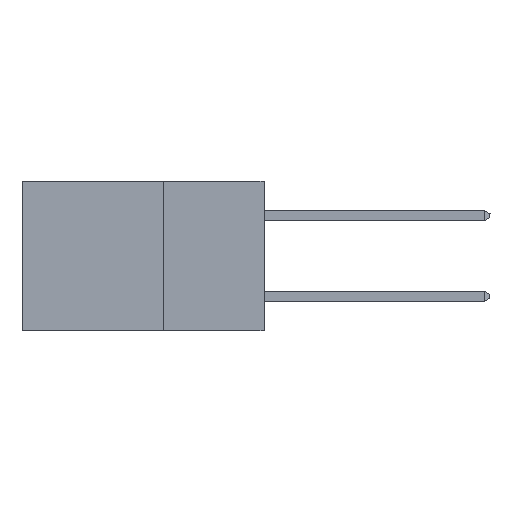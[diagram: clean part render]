
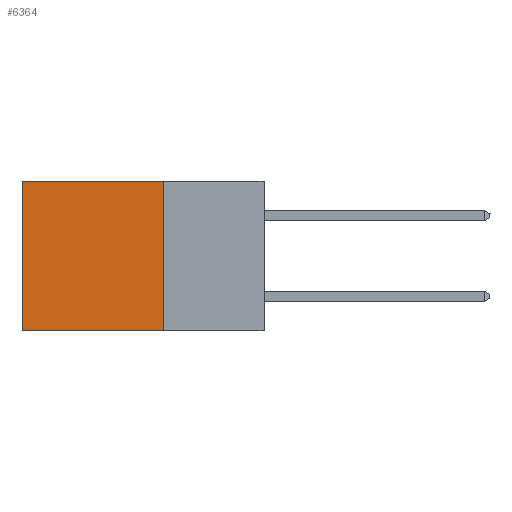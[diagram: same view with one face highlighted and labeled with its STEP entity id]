
A CAD part, left-side view. The second image highlights one B-rep face of the part: STEP entity #6364.
In plain terms, the highlighted planar face has unit normal (-1, 0, 0).
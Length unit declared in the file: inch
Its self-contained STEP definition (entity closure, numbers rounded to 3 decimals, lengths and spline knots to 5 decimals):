
#117 = CARTESIAN_POINT ( 'NONE',  ( 0.298, 0.6, 0. ) ) ;
#541 = CARTESIAN_POINT ( 'NONE',  ( 0.298, 0.25, 0. ) ) ;
#581 = DIRECTION ( 'NONE',  ( 1., 0., 0. ) ) ;
#1077 = DIRECTION ( 'NONE',  ( 0., 0., -1. ) ) ;
#1420 = EDGE_CURVE ( 'NONE', #4707, #4011, #1444, .T. ) ;
#1444 = LINE ( 'NONE', #8950, #5295 ) ;
#1672 = DIRECTION ( 'NONE',  ( 0., 1., 0. ) ) ;
#2638 = EDGE_LOOP ( 'NONE', ( #7657, #5121, #7415, #6482 ) ) ;
#3035 = DIRECTION ( 'NONE',  ( 0., 0., -1. ) ) ;
#3456 = DIRECTION ( 'NONE',  ( 0., 1., 0. ) ) ;
#3514 = VECTOR ( 'NONE', #3456, 39.37008 ) ;
#4011 = VERTEX_POINT ( 'NONE', #4131 ) ;
#4131 = CARTESIAN_POINT ( 'NONE',  ( 0.298, 0.25, -0.37 ) ) ;
#4133 = CARTESIAN_POINT ( 'NONE',  ( 0.298, 0.25, -0.37 ) ) ;
#4216 = VERTEX_POINT ( 'NONE', #6704 ) ;
#4707 = VERTEX_POINT ( 'NONE', #9770 ) ;
#4790 = VECTOR ( 'NONE', #1077, 39.37008 ) ;
#5121 = ORIENTED_EDGE ( 'NONE', *, *, #6681, .F. ) ;
#5295 = VECTOR ( 'NONE', #10662, 39.37008 ) ;
#5857 = EDGE_CURVE ( 'NONE', #4707, #9019, #9291, .T. ) ;
#6364 = ADVANCED_FACE ( 'NONE', ( #7934 ), #9168, .F. ) ;
#6453 = LINE ( 'NONE', #9165, #4790 ) ;
#6482 = ORIENTED_EDGE ( 'NONE', *, *, #5857, .T. ) ;
#6557 = VECTOR ( 'NONE', #1672, 39.37008 ) ;
#6681 = EDGE_CURVE ( 'NONE', #4011, #4216, #8730, .T. ) ;
#6704 = CARTESIAN_POINT ( 'NONE',  ( 0.298, 0.6, -0.37 ) ) ;
#7415 = ORIENTED_EDGE ( 'NONE', *, *, #1420, .F. ) ;
#7657 = ORIENTED_EDGE ( 'NONE', *, *, #11211, .T. ) ;
#7719 = AXIS2_PLACEMENT_3D ( 'NONE', #541, #581, #3035 ) ;
#7762 = CARTESIAN_POINT ( 'NONE',  ( 0.298, 0.25, 0. ) ) ;
#7934 = FACE_OUTER_BOUND ( 'NONE', #2638, .T. ) ;
#8730 = LINE ( 'NONE', #4133, #3514 ) ;
#8950 = CARTESIAN_POINT ( 'NONE',  ( 0.298, 0.25, 0. ) ) ;
#9019 = VERTEX_POINT ( 'NONE', #117 ) ;
#9165 = CARTESIAN_POINT ( 'NONE',  ( 0.298, 0.6, 0. ) ) ;
#9168 = PLANE ( 'NONE',  #7719 ) ;
#9291 = LINE ( 'NONE', #7762, #6557 ) ;
#9770 = CARTESIAN_POINT ( 'NONE',  ( 0.298, 0.25, 0. ) ) ;
#10662 = DIRECTION ( 'NONE',  ( 0., 0., -1. ) ) ;
#11211 = EDGE_CURVE ( 'NONE', #9019, #4216, #6453, .T. ) ;
